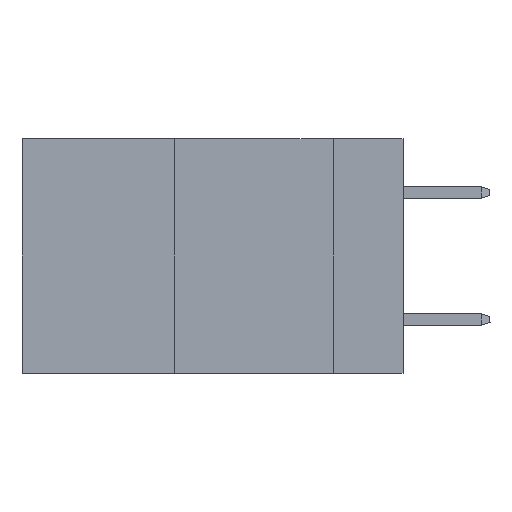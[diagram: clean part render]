
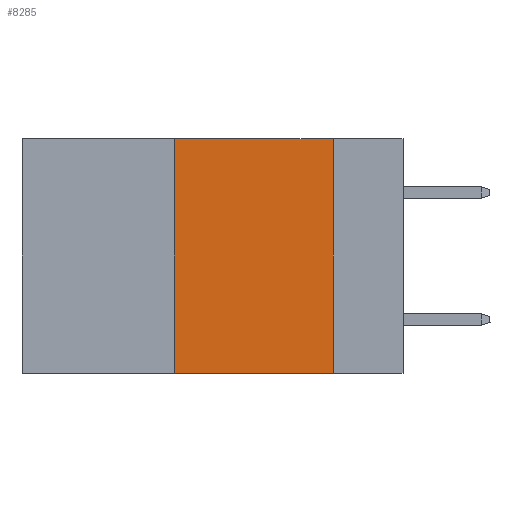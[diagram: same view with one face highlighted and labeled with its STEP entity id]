
A CAD part, left-side view. The second image highlights one B-rep face of the part: STEP entity #8285.
In plain terms, the highlighted planar face has unit normal (-1, 0, 0).
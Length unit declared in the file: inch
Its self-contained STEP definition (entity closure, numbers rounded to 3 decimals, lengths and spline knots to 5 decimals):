
#228 = CARTESIAN_POINT ( 'NONE',  ( 0., 0.6, 0. ) ) ;
#425 = CARTESIAN_POINT ( 'NONE',  ( 0., 0.36, -0.37 ) ) ;
#566 = FACE_OUTER_BOUND ( 'NONE', #15395, .T. ) ;
#702 = PLANE ( 'NONE',  #12040 ) ;
#2190 = ORIENTED_EDGE ( 'NONE', *, *, #7634, .T. ) ;
#2895 = DIRECTION ( 'NONE',  ( 0., 0., -1. ) ) ;
#4909 = EDGE_CURVE ( 'NONE', #11050, #23213, #17087, .T. ) ;
#5516 = CARTESIAN_POINT ( 'NONE',  ( 0., 0.36, 0. ) ) ;
#5800 = VERTEX_POINT ( 'NONE', #22412 ) ;
#6279 = VECTOR ( 'NONE', #17795, 39.37008 ) ;
#7547 = LINE ( 'NONE', #15987, #6279 ) ;
#7634 = EDGE_CURVE ( 'NONE', #20944, #5800, #13412, .T. ) ;
#8249 = DIRECTION ( 'NONE',  ( 0., -1., 0. ) ) ;
#8285 = ADVANCED_FACE ( 'NONE', ( #566 ), #702, .F. ) ;
#11050 = VERTEX_POINT ( 'NONE', #14924 ) ;
#11335 = CARTESIAN_POINT ( 'NONE',  ( 0., 0.6, 0. ) ) ;
#11904 = VECTOR ( 'NONE', #8249, 39.37008 ) ;
#11987 = LINE ( 'NONE', #5516, #13423 ) ;
#12040 = AXIS2_PLACEMENT_3D ( 'NONE', #11335, #23960, #2895 ) ;
#12687 = CARTESIAN_POINT ( 'NONE',  ( 0., 0.11, 0. ) ) ;
#12824 = EDGE_CURVE ( 'NONE', #23213, #5800, #7547, .T. ) ;
#13412 = LINE ( 'NONE', #24389, #15085 ) ;
#13423 = VECTOR ( 'NONE', #20446, 39.37008 ) ;
#14304 = ORIENTED_EDGE ( 'NONE', *, *, #4909, .F. ) ;
#14924 = CARTESIAN_POINT ( 'NONE',  ( 0., 0.36, 0. ) ) ;
#15085 = VECTOR ( 'NONE', #26189, 39.37008 ) ;
#15395 = EDGE_LOOP ( 'NONE', ( #26407, #14304, #25775, #2190 ) ) ;
#15987 = CARTESIAN_POINT ( 'NONE',  ( 0., 0.11, 0. ) ) ;
#17087 = LINE ( 'NONE', #228, #11904 ) ;
#17795 = DIRECTION ( 'NONE',  ( 0., 0., -1. ) ) ;
#17885 = EDGE_CURVE ( 'NONE', #20944, #11050, #11987, .T. ) ;
#20446 = DIRECTION ( 'NONE',  ( 0., 0., 1. ) ) ;
#20944 = VERTEX_POINT ( 'NONE', #425 ) ;
#22412 = CARTESIAN_POINT ( 'NONE',  ( 0., 0.11, -0.37 ) ) ;
#23213 = VERTEX_POINT ( 'NONE', #12687 ) ;
#23960 = DIRECTION ( 'NONE',  ( 1., 0., 0. ) ) ;
#24389 = CARTESIAN_POINT ( 'NONE',  ( 0., 0.6, -0.37 ) ) ;
#25775 = ORIENTED_EDGE ( 'NONE', *, *, #17885, .F. ) ;
#26189 = DIRECTION ( 'NONE',  ( 0., -1., 0. ) ) ;
#26407 = ORIENTED_EDGE ( 'NONE', *, *, #12824, .F. ) ;
